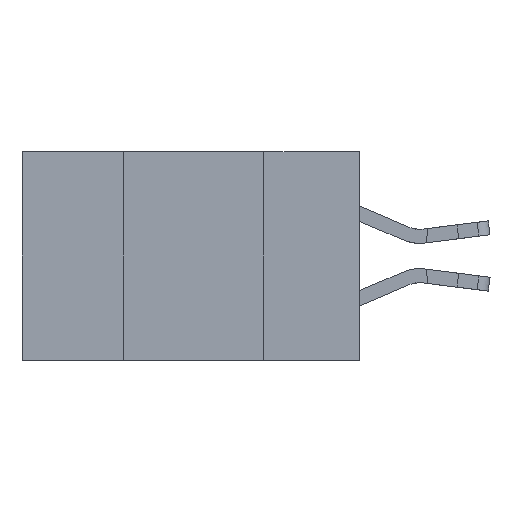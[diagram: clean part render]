
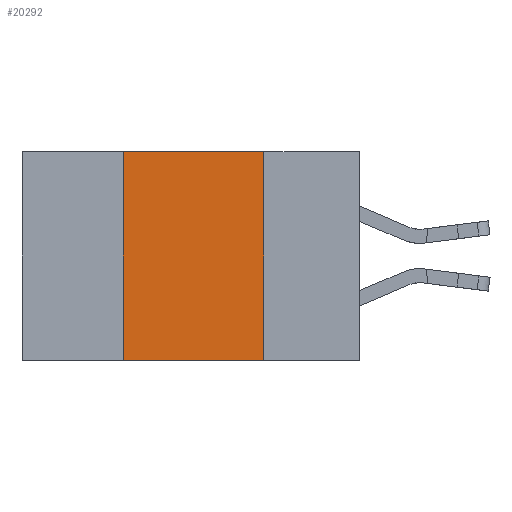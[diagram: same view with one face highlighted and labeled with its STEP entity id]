
A CAD part, left-side view. The second image highlights one B-rep face of the part: STEP entity #20292.
In plain terms, the highlighted planar face has unit normal (-1, 0, 0).
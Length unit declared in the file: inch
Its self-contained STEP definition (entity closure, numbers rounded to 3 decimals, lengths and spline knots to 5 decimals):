
#101 = CARTESIAN_POINT ( 'NONE',  ( 0., 0.6, 0. ) ) ;
#299 = VERTEX_POINT ( 'NONE', #23168 ) ;
#444 = FACE_OUTER_BOUND ( 'NONE', #17179, .T. ) ;
#1724 = CARTESIAN_POINT ( 'NONE',  ( 0., 0.42, 0. ) ) ;
#1890 = ORIENTED_EDGE ( 'NONE', *, *, #25750, .F. ) ;
#2183 = DIRECTION ( 'NONE',  ( 0., 0., -1. ) ) ;
#2939 = LINE ( 'NONE', #20844, #3649 ) ;
#3183 = ORIENTED_EDGE ( 'NONE', *, *, #7284, .F. ) ;
#3305 = LINE ( 'NONE', #14904, #11285 ) ;
#3649 = VECTOR ( 'NONE', #20945, 39.37008 ) ;
#4549 = LINE ( 'NONE', #1724, #26212 ) ;
#4927 = ORIENTED_EDGE ( 'NONE', *, *, #25460, .T. ) ;
#6468 = DIRECTION ( 'NONE',  ( 0., 0., 1. ) ) ;
#7284 = EDGE_CURVE ( 'NONE', #299, #28028, #14232, .T. ) ;
#8762 = DIRECTION ( 'NONE',  ( 0., -1., 0. ) ) ;
#10715 = AXIS2_PLACEMENT_3D ( 'NONE', #101, #24155, #15350 ) ;
#10802 = CARTESIAN_POINT ( 'NONE',  ( 0., 0.17, 0. ) ) ;
#11285 = VECTOR ( 'NONE', #8762, 39.37008 ) ;
#12440 = CARTESIAN_POINT ( 'NONE',  ( 0., 0.42, -0.37 ) ) ;
#13393 = PLANE ( 'NONE',  #10715 ) ;
#13739 = EDGE_CURVE ( 'NONE', #17784, #24110, #4549, .T. ) ;
#14232 = LINE ( 'NONE', #10802, #16712 ) ;
#14904 = CARTESIAN_POINT ( 'NONE',  ( 0., 0.6, -0.37 ) ) ;
#15350 = DIRECTION ( 'NONE',  ( 0., 0., -1. ) ) ;
#16712 = VECTOR ( 'NONE', #2183, 39.37008 ) ;
#17179 = EDGE_LOOP ( 'NONE', ( #3183, #1890, #20538, #4927 ) ) ;
#17784 = VERTEX_POINT ( 'NONE', #12440 ) ;
#20292 = ADVANCED_FACE ( 'NONE', ( #444 ), #13393, .F. ) ;
#20538 = ORIENTED_EDGE ( 'NONE', *, *, #13739, .F. ) ;
#20844 = CARTESIAN_POINT ( 'NONE',  ( 0., 0.6, 0. ) ) ;
#20945 = DIRECTION ( 'NONE',  ( 0., -1., 0. ) ) ;
#22297 = CARTESIAN_POINT ( 'NONE',  ( 0., 0.42, 0. ) ) ;
#23168 = CARTESIAN_POINT ( 'NONE',  ( 0., 0.17, 0. ) ) ;
#24110 = VERTEX_POINT ( 'NONE', #22297 ) ;
#24155 = DIRECTION ( 'NONE',  ( 1., 0., 0. ) ) ;
#24832 = CARTESIAN_POINT ( 'NONE',  ( 0., 0.17, -0.37 ) ) ;
#25460 = EDGE_CURVE ( 'NONE', #17784, #28028, #3305, .T. ) ;
#25750 = EDGE_CURVE ( 'NONE', #24110, #299, #2939, .T. ) ;
#26212 = VECTOR ( 'NONE', #6468, 39.37008 ) ;
#28028 = VERTEX_POINT ( 'NONE', #24832 ) ;
